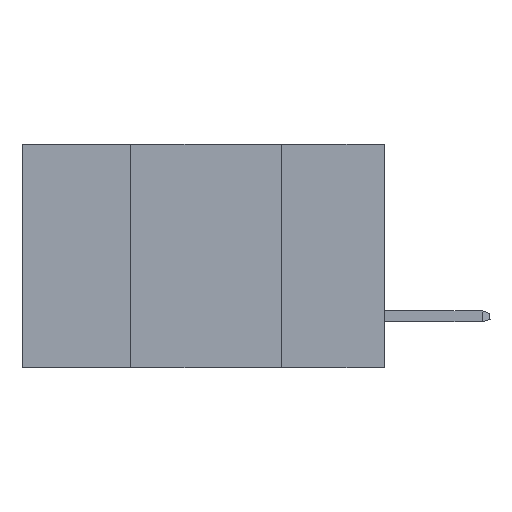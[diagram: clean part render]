
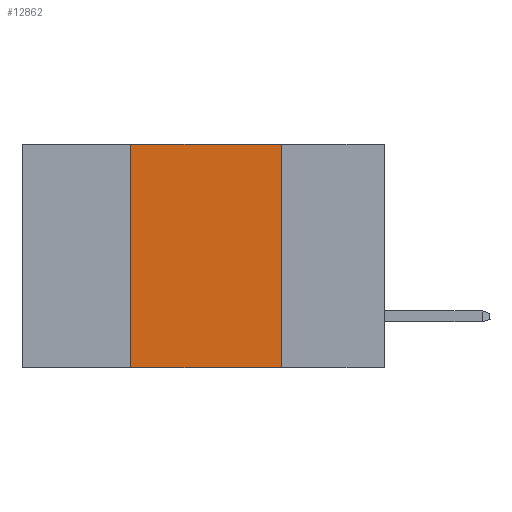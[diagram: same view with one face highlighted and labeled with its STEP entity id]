
A CAD part, left-side view. The second image highlights one B-rep face of the part: STEP entity #12862.
In plain terms, the highlighted planar face has unit normal (-1, 0, 0).
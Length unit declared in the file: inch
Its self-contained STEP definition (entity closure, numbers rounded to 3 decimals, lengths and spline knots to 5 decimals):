
#686 = ORIENTED_EDGE ( 'NONE', *, *, #5496, .F. ) ;
#1381 = VECTOR ( 'NONE', #9083, 39.37008 ) ;
#1710 = PLANE ( 'NONE',  #12557 ) ;
#2139 = CARTESIAN_POINT ( 'NONE',  ( 0., 0.42, -0.37 ) ) ;
#3055 = CARTESIAN_POINT ( 'NONE',  ( 0., 0.6, 0. ) ) ;
#4107 = LINE ( 'NONE', #6187, #12291 ) ;
#4199 = DIRECTION ( 'NONE',  ( 0., 0., -1. ) ) ;
#4245 = ORIENTED_EDGE ( 'NONE', *, *, #7782, .F. ) ;
#4274 = ORIENTED_EDGE ( 'NONE', *, *, #5924, .T. ) ;
#4488 = CARTESIAN_POINT ( 'NONE',  ( 0., 0.42, 0. ) ) ;
#4522 = LINE ( 'NONE', #4488, #1381 ) ;
#5031 = ORIENTED_EDGE ( 'NONE', *, *, #9493, .F. ) ;
#5088 = CARTESIAN_POINT ( 'NONE',  ( 0., 0.42, 0. ) ) ;
#5496 = EDGE_CURVE ( 'NONE', #12024, #15291, #4107, .T. ) ;
#5924 = EDGE_CURVE ( 'NONE', #10789, #15291, #11720, .T. ) ;
#6187 = CARTESIAN_POINT ( 'NONE',  ( 0., 0.17, 0. ) ) ;
#6447 = CARTESIAN_POINT ( 'NONE',  ( 0., 0.17, -0.37 ) ) ;
#6873 = DIRECTION ( 'NONE',  ( 0., -1., 0. ) ) ;
#6906 = CARTESIAN_POINT ( 'NONE',  ( 0., 0.17, 0. ) ) ;
#7782 = EDGE_CURVE ( 'NONE', #8550, #12024, #12755, .T. ) ;
#8550 = VERTEX_POINT ( 'NONE', #5088 ) ;
#8819 = VECTOR ( 'NONE', #10526, 39.37008 ) ;
#9083 = DIRECTION ( 'NONE',  ( 0., 0., 1. ) ) ;
#9264 = VECTOR ( 'NONE', #6873, 39.37008 ) ;
#9476 = EDGE_LOOP ( 'NONE', ( #686, #4245, #5031, #4274 ) ) ;
#9493 = EDGE_CURVE ( 'NONE', #10789, #8550, #4522, .T. ) ;
#10526 = DIRECTION ( 'NONE',  ( 0., -1., 0. ) ) ;
#10789 = VERTEX_POINT ( 'NONE', #2139 ) ;
#11720 = LINE ( 'NONE', #11861, #9264 ) ;
#11861 = CARTESIAN_POINT ( 'NONE',  ( 0., 0.6, -0.37 ) ) ;
#12024 = VERTEX_POINT ( 'NONE', #6906 ) ;
#12291 = VECTOR ( 'NONE', #13268, 39.37008 ) ;
#12557 = AXIS2_PLACEMENT_3D ( 'NONE', #3055, #13759, #4199 ) ;
#12755 = LINE ( 'NONE', #15259, #8819 ) ;
#12862 = ADVANCED_FACE ( 'NONE', ( #14113 ), #1710, .F. ) ;
#13268 = DIRECTION ( 'NONE',  ( 0., 0., -1. ) ) ;
#13759 = DIRECTION ( 'NONE',  ( 1., 0., 0. ) ) ;
#14113 = FACE_OUTER_BOUND ( 'NONE', #9476, .T. ) ;
#15259 = CARTESIAN_POINT ( 'NONE',  ( 0., 0.6, 0. ) ) ;
#15291 = VERTEX_POINT ( 'NONE', #6447 ) ;
